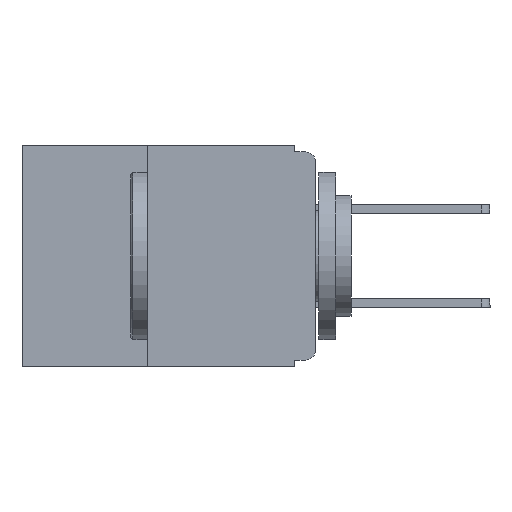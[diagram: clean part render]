
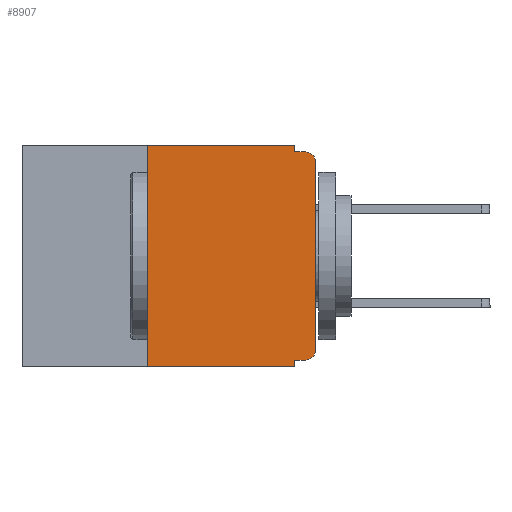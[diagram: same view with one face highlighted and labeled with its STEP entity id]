
A CAD part, left-side view. The second image highlights one B-rep face of the part: STEP entity #8907.
In plain terms, the highlighted planar face has unit normal (-1, 0, 0).
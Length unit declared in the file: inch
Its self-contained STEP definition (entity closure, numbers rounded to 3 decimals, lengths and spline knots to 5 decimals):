
#177 = CARTESIAN_POINT ( 'NONE',  ( 0., 0.031, -0.33 ) ) ;
#590 = AXIS2_PLACEMENT_3D ( 'NONE', #6749, #4517, #11113 ) ;
#1481 = EDGE_CURVE ( 'NONE', #25940, #28060, #25063, .T. ) ;
#1676 = DIRECTION ( 'NONE',  ( -1., 0., 0. ) ) ;
#2133 = CARTESIAN_POINT ( 'NONE',  ( 0., 0.25, -0.33 ) ) ;
#2185 = VERTEX_POINT ( 'NONE', #9238 ) ;
#2250 = CARTESIAN_POINT ( 'NONE',  ( 0., 0.437, 0. ) ) ;
#2423 = EDGE_CURVE ( 'NONE', #14557, #3387, #23028, .T. ) ;
#2610 = VECTOR ( 'NONE', #16336, 39.37008 ) ;
#3387 = VERTEX_POINT ( 'NONE', #15750 ) ;
#4517 = DIRECTION ( 'NONE',  ( 1., 0., 0. ) ) ;
#4757 = LINE ( 'NONE', #177, #26420 ) ;
#4932 = VERTEX_POINT ( 'NONE', #23146 ) ;
#5719 = VECTOR ( 'NONE', #12914, 39.37008 ) ;
#6466 = AXIS2_PLACEMENT_3D ( 'NONE', #9189, #24307, #11365 ) ;
#6749 = CARTESIAN_POINT ( 'NONE',  ( 0., 0.437, 0. ) ) ;
#6840 = ORIENTED_EDGE ( 'NONE', *, *, #27298, .T. ) ;
#8270 = CARTESIAN_POINT ( 'NONE',  ( 0., 0., -0.01 ) ) ;
#8639 = EDGE_CURVE ( 'NONE', #2185, #14241, #11555, .T. ) ;
#8907 = ADVANCED_FACE ( 'NONE', ( #10502 ), #24050, .F. ) ;
#9189 = CARTESIAN_POINT ( 'NONE',  ( 0., 0.015, -0.305 ) ) ;
#9238 = CARTESIAN_POINT ( 'NONE',  ( 0., 0.015, -0.32 ) ) ;
#9514 = CARTESIAN_POINT ( 'NONE',  ( 0., 0.25, 0. ) ) ;
#10255 = ORIENTED_EDGE ( 'NONE', *, *, #20179, .T. ) ;
#10502 = FACE_OUTER_BOUND ( 'NONE', #14934, .T. ) ;
#11113 = DIRECTION ( 'NONE',  ( 0., 0., -1. ) ) ;
#11365 = DIRECTION ( 'NONE',  ( 0., 0., -1. ) ) ;
#11404 = CARTESIAN_POINT ( 'NONE',  ( 0., 0.25, -0.33 ) ) ;
#11555 = LINE ( 'NONE', #14555, #22387 ) ;
#12481 = EDGE_CURVE ( 'NONE', #14448, #14200, #17859, .T. ) ;
#12612 = DIRECTION ( 'NONE',  ( 0., -1., 0. ) ) ;
#12687 = VECTOR ( 'NONE', #12612, 39.37008 ) ;
#12914 = DIRECTION ( 'NONE',  ( 0., -1., 0. ) ) ;
#13445 = DIRECTION ( 'NONE',  ( 0., 0., -1. ) ) ;
#13518 = CARTESIAN_POINT ( 'NONE',  ( 0., 0.031, -0.01 ) ) ;
#13919 = EDGE_CURVE ( 'NONE', #14241, #28060, #4757, .T. ) ;
#14200 = VERTEX_POINT ( 'NONE', #27586 ) ;
#14241 = VERTEX_POINT ( 'NONE', #19379 ) ;
#14448 = VERTEX_POINT ( 'NONE', #13518 ) ;
#14555 = CARTESIAN_POINT ( 'NONE',  ( 0., 0., -0.32 ) ) ;
#14557 = VERTEX_POINT ( 'NONE', #9514 ) ;
#14886 = CARTESIAN_POINT ( 'NONE',  ( 0., 0.015, -0.025 ) ) ;
#14893 = ORIENTED_EDGE ( 'NONE', *, *, #28003, .F. ) ;
#14934 = EDGE_LOOP ( 'NONE', ( #6840, #10255, #21476, #27073, #24114, #14893, #19261, #19663, #23698, #24007 ) ) ;
#14992 = VECTOR ( 'NONE', #24538, 39.37008 ) ;
#15750 = CARTESIAN_POINT ( 'NONE',  ( 0., 0.031, 0. ) ) ;
#16086 = CARTESIAN_POINT ( 'NONE',  ( 0., 0., 0. ) ) ;
#16336 = DIRECTION ( 'NONE',  ( 0., -1., 0. ) ) ;
#17093 = DIRECTION ( 'NONE',  ( 0., 0., -1. ) ) ;
#17158 = EDGE_CURVE ( 'NONE', #2185, #18121, #21127, .T. ) ;
#17698 = VECTOR ( 'NONE', #20369, 39.37008 ) ;
#17859 = LINE ( 'NONE', #8270, #12687 ) ;
#17874 = EDGE_CURVE ( 'NONE', #3387, #14448, #25731, .T. ) ;
#18121 = VERTEX_POINT ( 'NONE', #18975 ) ;
#18375 = LINE ( 'NONE', #16086, #17698 ) ;
#18692 = LINE ( 'NONE', #11404, #27925 ) ;
#18975 = CARTESIAN_POINT ( 'NONE',  ( 0., 0., -0.305 ) ) ;
#19261 = ORIENTED_EDGE ( 'NONE', *, *, #1481, .T. ) ;
#19379 = CARTESIAN_POINT ( 'NONE',  ( 0., 0.031, -0.32 ) ) ;
#19663 = ORIENTED_EDGE ( 'NONE', *, *, #13919, .F. ) ;
#20179 = EDGE_CURVE ( 'NONE', #4932, #14200, #22276, .T. ) ;
#20369 = DIRECTION ( 'NONE',  ( 0., 0., 1. ) ) ;
#21127 = CIRCLE ( 'NONE', #6466, 0.015 ) ;
#21414 = AXIS2_PLACEMENT_3D ( 'NONE', #14886, #1676, #17093 ) ;
#21476 = ORIENTED_EDGE ( 'NONE', *, *, #12481, .F. ) ;
#21914 = CARTESIAN_POINT ( 'NONE',  ( 0., 0.437, -0.33 ) ) ;
#22209 = DIRECTION ( 'NONE',  ( 0., 0., 1. ) ) ;
#22276 = CIRCLE ( 'NONE', #21414, 0.015 ) ;
#22387 = VECTOR ( 'NONE', #23219, 39.37008 ) ;
#22408 = CARTESIAN_POINT ( 'NONE',  ( 0., 0.031, 0. ) ) ;
#23028 = LINE ( 'NONE', #2250, #5719 ) ;
#23146 = CARTESIAN_POINT ( 'NONE',  ( 0., 0., -0.025 ) ) ;
#23219 = DIRECTION ( 'NONE',  ( 0., 1., 0. ) ) ;
#23698 = ORIENTED_EDGE ( 'NONE', *, *, #8639, .F. ) ;
#24007 = ORIENTED_EDGE ( 'NONE', *, *, #17158, .T. ) ;
#24050 = PLANE ( 'NONE',  #590 ) ;
#24114 = ORIENTED_EDGE ( 'NONE', *, *, #2423, .F. ) ;
#24307 = DIRECTION ( 'NONE',  ( -1., 0., 0. ) ) ;
#24538 = DIRECTION ( 'NONE',  ( 0., 0., -1. ) ) ;
#24608 = CARTESIAN_POINT ( 'NONE',  ( 0., 0.031, -0.33 ) ) ;
#25063 = LINE ( 'NONE', #21914, #2610 ) ;
#25731 = LINE ( 'NONE', #22408, #14992 ) ;
#25940 = VERTEX_POINT ( 'NONE', #2133 ) ;
#26420 = VECTOR ( 'NONE', #13445, 39.37008 ) ;
#27073 = ORIENTED_EDGE ( 'NONE', *, *, #17874, .F. ) ;
#27298 = EDGE_CURVE ( 'NONE', #18121, #4932, #18375, .T. ) ;
#27586 = CARTESIAN_POINT ( 'NONE',  ( 0., 0.015, -0.01 ) ) ;
#27925 = VECTOR ( 'NONE', #22209, 39.37008 ) ;
#28003 = EDGE_CURVE ( 'NONE', #25940, #14557, #18692, .T. ) ;
#28060 = VERTEX_POINT ( 'NONE', #24608 ) ;
